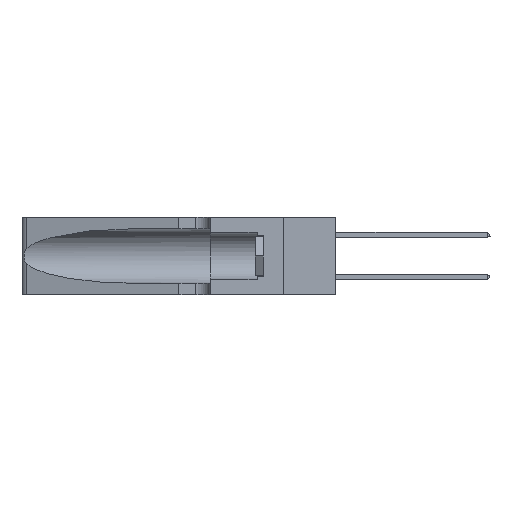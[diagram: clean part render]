
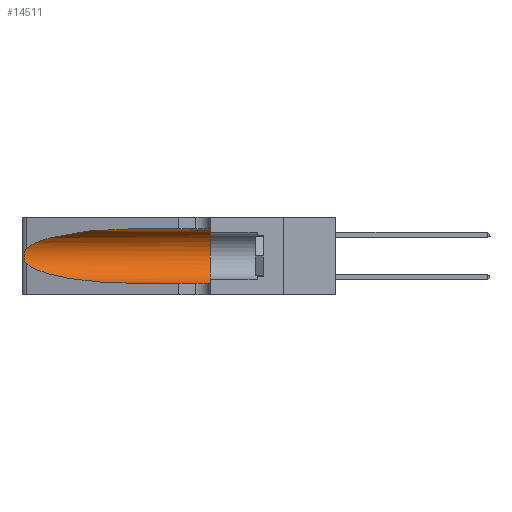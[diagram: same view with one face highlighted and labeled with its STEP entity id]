
A CAD part, left-side view. The second image highlights one B-rep face of the part: STEP entity #14511.
In plain terms, the highlighted cylindrical face has radius 3.308 mm (diameter 6.617 mm), a partial arc.
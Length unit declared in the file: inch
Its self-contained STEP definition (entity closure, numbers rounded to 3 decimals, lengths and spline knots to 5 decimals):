
#511 = CARTESIAN_POINT ( 'NONE',  ( 0.25789, 1.23486, 0.15765 ) ) ;
#1443 = AXIS2_PLACEMENT_3D ( 'NONE', #13147, #30565, #21883 ) ;
#3065 = VECTOR ( 'NONE', #23263, 39.37008 ) ;
#3351 =( BOUNDED_CURVE ( )  B_SPLINE_CURVE ( 3, ( #18569, #9714, #9845, #27621 ),
 .UNSPECIFIED., .F., .F. ) 
 B_SPLINE_CURVE_WITH_KNOTS ( ( 4, 4 ),
 ( 3.44316, 4.71239 ),
 .UNSPECIFIED. ) 
 CURVE ( )  GEOMETRIC_REPRESENTATION_ITEM ( )  RATIONAL_B_SPLINE_CURVE ( ( 1., 0.87, 0.87, 1. ) ) 
 REPRESENTATION_ITEM ( '' )  );
#3648 = VERTEX_POINT ( 'NONE', #20704 ) ;
#3734 = EDGE_CURVE ( 'NONE', #36361, #14221, #23297, .T. ) ;
#4868 = AXIS2_PLACEMENT_3D ( 'NONE', #16723, #17259, #8370 ) ;
#4950 = VERTEX_POINT ( 'NONE', #16909 ) ;
#4994 = DIRECTION ( 'NONE',  ( 0., -1., 0. ) ) ;
#5647 = CARTESIAN_POINT ( 'NONE',  ( 0.25487, 1.22718, 0.14631 ) ) ;
#6177 =( BOUNDED_CURVE ( )  B_SPLINE_CURVE ( 3, ( #7822, #16572, #34242, #16313 ),
 .UNSPECIFIED., .F., .F. ) 
 B_SPLINE_CURVE_WITH_KNOTS ( ( 4, 4 ),
 ( 1.5708, 2.84003 ),
 .UNSPECIFIED. ) 
 CURVE ( )  GEOMETRIC_REPRESENTATION_ITEM ( )  RATIONAL_B_SPLINE_CURVE ( ( 1., 0.87, 0.87, 1. ) ) 
 REPRESENTATION_ITEM ( '' )  );
#6275 = ORIENTED_EDGE ( 'NONE', *, *, #22068, .F. ) ;
#7822 = CARTESIAN_POINT ( 'NONE',  ( 0.1305, 0.72297, 0.31525 ) ) ;
#8370 = DIRECTION ( 'NONE',  ( 0., 0., 1. ) ) ;
#9001 = B_SPLINE_CURVE_WITH_KNOTS ( 'NONE', 3,
 ( #15625, #27480, #20218, #32388, #23576, #36242, #27148, #27321, #16090, #37655, #511, #26064, #29640, #29042 ),
 .UNSPECIFIED., .F., .F.,
 ( 4, 2, 2, 2, 2, 2, 4 ),
 ( 0., 0.00027, 0.00053, 0.00107, 0.0016, 0.00187, 0.00214 ),
 .UNSPECIFIED. ) ;
#9317 = ORIENTED_EDGE ( 'NONE', *, *, #11178, .F. ) ;
#9649 = FACE_OUTER_BOUND ( 'NONE', #18211, .T. ) ;
#9714 = CARTESIAN_POINT ( 'NONE',  ( 0.2373, 1.15595, 0.08982 ) ) ;
#9845 = CARTESIAN_POINT ( 'NONE',  ( 0.18966, 0.96281, 0.05475 ) ) ;
#10517 = ORIENTED_EDGE ( 'NONE', *, *, #23195, .T. ) ;
#10533 = CIRCLE ( 'NONE', #4868, 0.13025 ) ;
#11178 = EDGE_CURVE ( 'NONE', #3648, #14221, #10533, .T. ) ;
#11944 = ORIENTED_EDGE ( 'NONE', *, *, #25186, .T. ) ;
#13147 = CARTESIAN_POINT ( 'NONE',  ( 0.1305, 1.61858, 0.185 ) ) ;
#14221 = VERTEX_POINT ( 'NONE', #17071 ) ;
#14511 = ADVANCED_FACE ( 'NONE', ( #9649 ), #36889, .F. ) ;
#14965 = ORIENTED_EDGE ( 'NONE', *, *, #29941, .T. ) ;
#15625 = CARTESIAN_POINT ( 'NONE',  ( 0.25487, 1.22718, 0.22369 ) ) ;
#16090 = CARTESIAN_POINT ( 'NONE',  ( 0.26017, 1.23833, 0.17102 ) ) ;
#16313 = CARTESIAN_POINT ( 'NONE',  ( 0.25487, 1.22718, 0.22369 ) ) ;
#16572 = CARTESIAN_POINT ( 'NONE',  ( 0.18966, 0.96281, 0.31525 ) ) ;
#16723 = CARTESIAN_POINT ( 'NONE',  ( 0.1305, 0.35, 0.185 ) ) ;
#16909 = CARTESIAN_POINT ( 'NONE',  ( 0.25487, 1.22718, 0.22369 ) ) ;
#17071 = CARTESIAN_POINT ( 'NONE',  ( 0.1305, 0.35, 0.05475 ) ) ;
#17259 = DIRECTION ( 'NONE',  ( 0., 1., 0. ) ) ;
#18211 = EDGE_LOOP ( 'NONE', ( #11944, #10517, #14965, #20155, #9317, #6275 ) ) ;
#18569 = CARTESIAN_POINT ( 'NONE',  ( 0.25487, 1.22718, 0.14631 ) ) ;
#20155 = ORIENTED_EDGE ( 'NONE', *, *, #3734, .T. ) ;
#20218 = CARTESIAN_POINT ( 'NONE',  ( 0.25639, 1.23184, 0.21858 ) ) ;
#20704 = CARTESIAN_POINT ( 'NONE',  ( 0.1305, 0.35, 0.31525 ) ) ;
#21085 = CARTESIAN_POINT ( 'NONE',  ( 0.1305, 0.72297, 0.05475 ) ) ;
#21883 = DIRECTION ( 'NONE',  ( 0., 0., -1. ) ) ;
#22068 = EDGE_CURVE ( 'NONE', #22745, #3648, #30852, .T. ) ;
#22551 = VERTEX_POINT ( 'NONE', #5647 ) ;
#22745 = VERTEX_POINT ( 'NONE', #36288 ) ;
#23195 = EDGE_CURVE ( 'NONE', #4950, #22551, #9001, .T. ) ;
#23263 = DIRECTION ( 'NONE',  ( 0., -1., 0. ) ) ;
#23297 = LINE ( 'NONE', #26112, #3065 ) ;
#23576 = CARTESIAN_POINT ( 'NONE',  ( 0.25854, 1.2359, 0.20912 ) ) ;
#25186 = EDGE_CURVE ( 'NONE', #22745, #4950, #6177, .T. ) ;
#25779 = VECTOR ( 'NONE', #4994, 39.37008 ) ;
#26064 = CARTESIAN_POINT ( 'NONE',  ( 0.25639, 1.23186, 0.15144 ) ) ;
#26112 = CARTESIAN_POINT ( 'NONE',  ( 0.1305, 1.61858, 0.05475 ) ) ;
#27148 = CARTESIAN_POINT ( 'NONE',  ( 0.26075, 1.23896, 0.19203 ) ) ;
#27321 = CARTESIAN_POINT ( 'NONE',  ( 0.26075, 1.23896, 0.178 ) ) ;
#27480 = CARTESIAN_POINT ( 'NONE',  ( 0.25555, 1.22994, 0.2215 ) ) ;
#27621 = CARTESIAN_POINT ( 'NONE',  ( 0.1305, 0.72297, 0.05475 ) ) ;
#29042 = CARTESIAN_POINT ( 'NONE',  ( 0.25487, 1.22718, 0.14631 ) ) ;
#29640 = CARTESIAN_POINT ( 'NONE',  ( 0.25555, 1.22993, 0.14849 ) ) ;
#29941 = EDGE_CURVE ( 'NONE', #22551, #36361, #3351, .T. ) ;
#30565 = DIRECTION ( 'NONE',  ( 0., -1., 0. ) ) ;
#30852 = LINE ( 'NONE', #37333, #25779 ) ;
#32388 = CARTESIAN_POINT ( 'NONE',  ( 0.25787, 1.23484, 0.2124 ) ) ;
#34242 = CARTESIAN_POINT ( 'NONE',  ( 0.2373, 1.15595, 0.28018 ) ) ;
#36242 = CARTESIAN_POINT ( 'NONE',  ( 0.26018, 1.23835, 0.19895 ) ) ;
#36288 = CARTESIAN_POINT ( 'NONE',  ( 0.1305, 0.72297, 0.31525 ) ) ;
#36361 = VERTEX_POINT ( 'NONE', #21085 ) ;
#36889 = CYLINDRICAL_SURFACE ( 'NONE', #1443, 0.13025 ) ;
#37333 = CARTESIAN_POINT ( 'NONE',  ( 0.1305, 1.61858, 0.31525 ) ) ;
#37655 = CARTESIAN_POINT ( 'NONE',  ( 0.25856, 1.23593, 0.16098 ) ) ;
